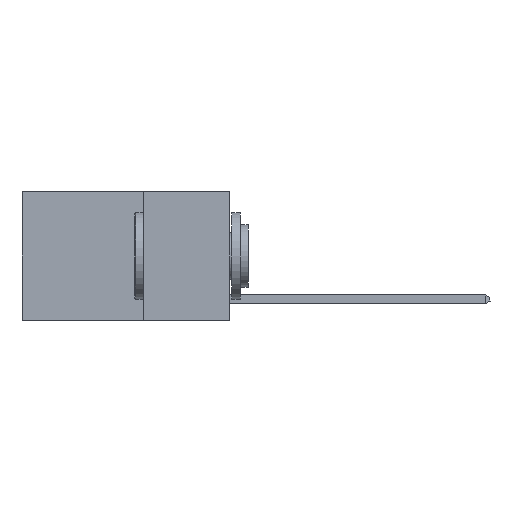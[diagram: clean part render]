
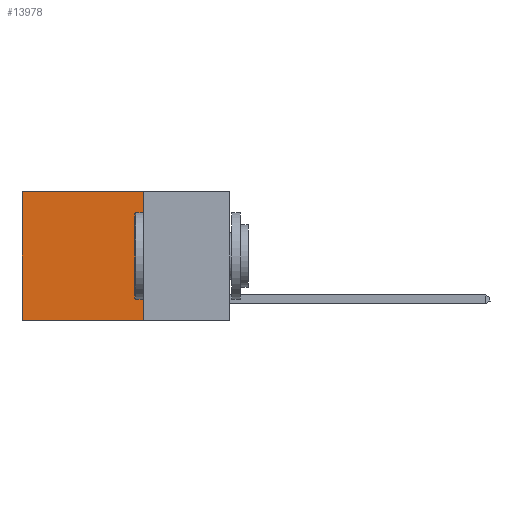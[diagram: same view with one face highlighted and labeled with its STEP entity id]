
A CAD part, left-side view. The second image highlights one B-rep face of the part: STEP entity #13978.
In plain terms, the highlighted planar face has unit normal (-1, 0, 0).
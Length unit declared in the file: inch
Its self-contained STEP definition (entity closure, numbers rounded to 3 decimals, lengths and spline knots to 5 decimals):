
#623 = DIRECTION ( 'NONE',  ( 0., 1., 0. ) ) ;
#996 = FACE_OUTER_BOUND ( 'NONE', #5266, .T. ) ;
#1022 = LINE ( 'NONE', #1137, #6380 ) ;
#1137 = CARTESIAN_POINT ( 'NONE',  ( 0.2625, 0.25, 0. ) ) ;
#2641 = CARTESIAN_POINT ( 'NONE',  ( 0.2625, 0.6, 0. ) ) ;
#2863 = DIRECTION ( 'NONE',  ( 0., 0., -1. ) ) ;
#4482 = DIRECTION ( 'NONE',  ( 0., 0., -1. ) ) ;
#5266 = EDGE_LOOP ( 'NONE', ( #20394, #19563, #15727, #20431 ) ) ;
#5351 = DIRECTION ( 'NONE',  ( 0., 0., -1. ) ) ;
#6380 = VECTOR ( 'NONE', #20387, 39.37008 ) ;
#6494 = CARTESIAN_POINT ( 'NONE',  ( 0.2625, 0.25, 0. ) ) ;
#6834 = VERTEX_POINT ( 'NONE', #6494 ) ;
#6982 = EDGE_CURVE ( 'NONE', #6834, #19005, #15710, .T. ) ;
#7719 = PLANE ( 'NONE',  #22504 ) ;
#8018 = CARTESIAN_POINT ( 'NONE',  ( 0.2625, 0.25, -0.37 ) ) ;
#8877 = VERTEX_POINT ( 'NONE', #18346 ) ;
#8969 = VECTOR ( 'NONE', #2863, 39.37008 ) ;
#10139 = CARTESIAN_POINT ( 'NONE',  ( 0.2625, 0.25, -0.37 ) ) ;
#11080 = VECTOR ( 'NONE', #623, 39.37008 ) ;
#12233 = CARTESIAN_POINT ( 'NONE',  ( 0.2625, 0.25, 0. ) ) ;
#13978 = ADVANCED_FACE ( 'NONE', ( #996 ), #7719, .F. ) ;
#14019 = CARTESIAN_POINT ( 'NONE',  ( 0.2625, 0.6, 0. ) ) ;
#15710 = LINE ( 'NONE', #12233, #17375 ) ;
#15727 = ORIENTED_EDGE ( 'NONE', *, *, #6982, .F. ) ;
#16812 = CARTESIAN_POINT ( 'NONE',  ( 0.2625, 0.25, 0. ) ) ;
#17144 = VERTEX_POINT ( 'NONE', #14019 ) ;
#17375 = VECTOR ( 'NONE', #5351, 39.37008 ) ;
#18346 = CARTESIAN_POINT ( 'NONE',  ( 0.2625, 0.6, -0.37 ) ) ;
#18375 = LINE ( 'NONE', #8018, #11080 ) ;
#18662 = LINE ( 'NONE', #2641, #8969 ) ;
#19005 = VERTEX_POINT ( 'NONE', #10139 ) ;
#19563 = ORIENTED_EDGE ( 'NONE', *, *, #19777, .F. ) ;
#19777 = EDGE_CURVE ( 'NONE', #19005, #8877, #18375, .T. ) ;
#20387 = DIRECTION ( 'NONE',  ( 0., 1., 0. ) ) ;
#20394 = ORIENTED_EDGE ( 'NONE', *, *, #22359, .T. ) ;
#20431 = ORIENTED_EDGE ( 'NONE', *, *, #22307, .T. ) ;
#21772 = DIRECTION ( 'NONE',  ( 1., 0., 0. ) ) ;
#22307 = EDGE_CURVE ( 'NONE', #6834, #17144, #1022, .T. ) ;
#22359 = EDGE_CURVE ( 'NONE', #17144, #8877, #18662, .T. ) ;
#22504 = AXIS2_PLACEMENT_3D ( 'NONE', #16812, #21772, #4482 ) ;
